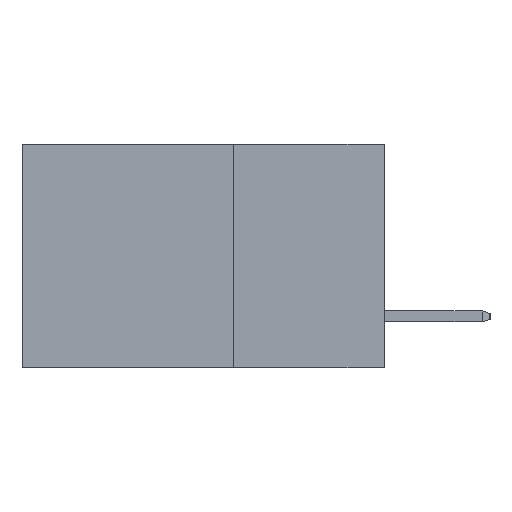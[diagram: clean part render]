
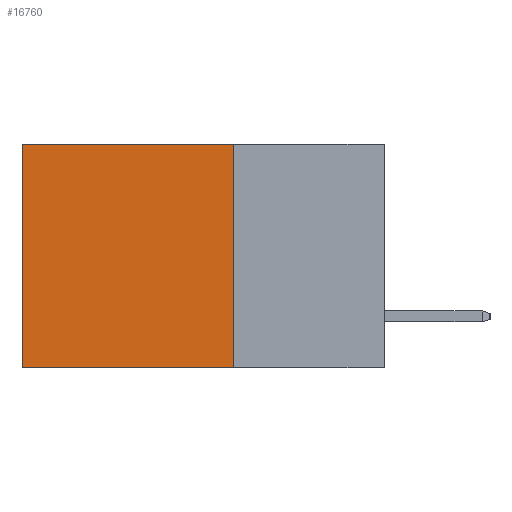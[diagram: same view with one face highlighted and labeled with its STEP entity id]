
A CAD part, left-side view. The second image highlights one B-rep face of the part: STEP entity #16760.
In plain terms, the highlighted planar face has unit normal (-1, 0, 0).
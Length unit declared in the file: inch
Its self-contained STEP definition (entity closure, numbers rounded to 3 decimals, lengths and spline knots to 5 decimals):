
#680 = DIRECTION ( 'NONE',  ( 0., 1., 0. ) ) ;
#758 = EDGE_CURVE ( 'NONE', #3117, #2033, #9352, .T. ) ;
#2033 = VERTEX_POINT ( 'NONE', #4316 ) ;
#2801 = VERTEX_POINT ( 'NONE', #9316 ) ;
#3117 = VERTEX_POINT ( 'NONE', #18691 ) ;
#4316 = CARTESIAN_POINT ( 'NONE',  ( 0.2615, 0.6, -0.37 ) ) ;
#4398 = ORIENTED_EDGE ( 'NONE', *, *, #15571, .T. ) ;
#4721 = AXIS2_PLACEMENT_3D ( 'NONE', #14993, #6441, #16365 ) ;
#4872 = VERTEX_POINT ( 'NONE', #9754 ) ;
#4998 = ORIENTED_EDGE ( 'NONE', *, *, #14995, .F. ) ;
#5302 = DIRECTION ( 'NONE',  ( 0., 1., 0. ) ) ;
#5568 = FACE_OUTER_BOUND ( 'NONE', #17725, .T. ) ;
#6276 = ORIENTED_EDGE ( 'NONE', *, *, #16556, .F. ) ;
#6441 = DIRECTION ( 'NONE',  ( 1., 0., 0. ) ) ;
#6721 = CARTESIAN_POINT ( 'NONE',  ( 0.2615, 0.25, 0. ) ) ;
#7409 = CARTESIAN_POINT ( 'NONE',  ( 0.2615, 0.25, -0.37 ) ) ;
#8869 = DIRECTION ( 'NONE',  ( 0., 0., -1. ) ) ;
#9316 = CARTESIAN_POINT ( 'NONE',  ( 0.2615, 0.25, 0. ) ) ;
#9352 = LINE ( 'NONE', #9705, #16384 ) ;
#9663 = DIRECTION ( 'NONE',  ( 0., 0., -1. ) ) ;
#9705 = CARTESIAN_POINT ( 'NONE',  ( 0.2615, 0.6, -0.37 ) ) ;
#9754 = CARTESIAN_POINT ( 'NONE',  ( 0.2615, 0.25, -0.37 ) ) ;
#10044 = ORIENTED_EDGE ( 'NONE', *, *, #758, .T. ) ;
#12012 = VECTOR ( 'NONE', #5302, 39.37008 ) ;
#12447 = LINE ( 'NONE', #18115, #12012 ) ;
#12452 = LINE ( 'NONE', #6721, #15668 ) ;
#13629 = PLANE ( 'NONE',  #4721 ) ;
#13939 = VECTOR ( 'NONE', #8869, 39.37008 ) ;
#14993 = CARTESIAN_POINT ( 'NONE',  ( 0.2615, 0.25, -0.37 ) ) ;
#14995 = EDGE_CURVE ( 'NONE', #4872, #2033, #12447, .T. ) ;
#15571 = EDGE_CURVE ( 'NONE', #2801, #3117, #12452, .T. ) ;
#15668 = VECTOR ( 'NONE', #680, 39.37008 ) ;
#16365 = DIRECTION ( 'NONE',  ( 0., 0., -1. ) ) ;
#16384 = VECTOR ( 'NONE', #9663, 39.37008 ) ;
#16556 = EDGE_CURVE ( 'NONE', #2801, #4872, #17133, .T. ) ;
#16760 = ADVANCED_FACE ( 'NONE', ( #5568 ), #13629, .F. ) ;
#17133 = LINE ( 'NONE', #7409, #13939 ) ;
#17725 = EDGE_LOOP ( 'NONE', ( #10044, #4998, #6276, #4398 ) ) ;
#18115 = CARTESIAN_POINT ( 'NONE',  ( 0.2615, 0.25, -0.37 ) ) ;
#18691 = CARTESIAN_POINT ( 'NONE',  ( 0.2615, 0.6, 0. ) ) ;
